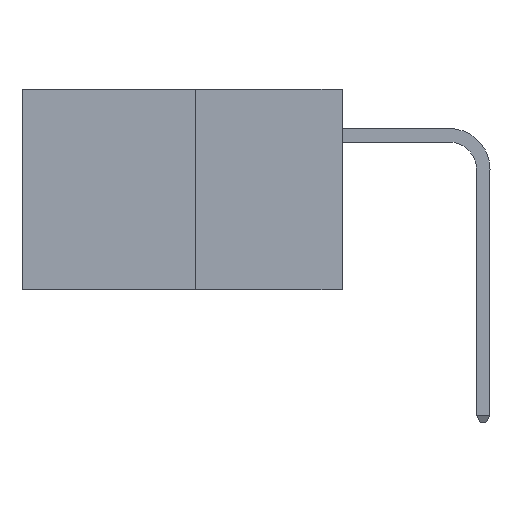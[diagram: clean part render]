
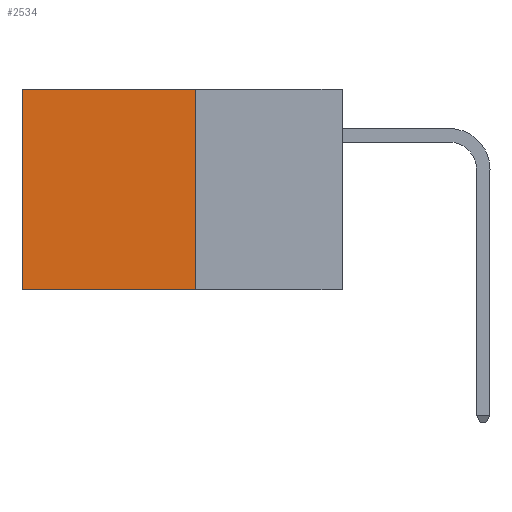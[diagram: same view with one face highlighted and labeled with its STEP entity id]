
A CAD part, left-side view. The second image highlights one B-rep face of the part: STEP entity #2534.
In plain terms, the highlighted planar face has unit normal (-1, 0, 0).
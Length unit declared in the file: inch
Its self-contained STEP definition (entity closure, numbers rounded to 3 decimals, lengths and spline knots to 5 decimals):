
#560 = EDGE_CURVE ( 'NONE', #17153, #22461, #20241, .T. ) ;
#880 = CARTESIAN_POINT ( 'NONE',  ( 0.277, 0.27, 0. ) ) ;
#1325 = VERTEX_POINT ( 'NONE', #22698 ) ;
#2214 = DIRECTION ( 'NONE',  ( 0., 0., -1. ) ) ;
#2436 = LINE ( 'NONE', #23840, #7656 ) ;
#2511 = DIRECTION ( 'NONE',  ( 1., 0., 0. ) ) ;
#2534 = ADVANCED_FACE ( 'NONE', ( #10246 ), #4251, .F. ) ;
#2813 = CARTESIAN_POINT ( 'NONE',  ( 0.277, 0.27, -0.37 ) ) ;
#4251 = PLANE ( 'NONE',  #25468 ) ;
#4839 = EDGE_LOOP ( 'NONE', ( #19494, #11584, #23456, #14546 ) ) ;
#6558 = DIRECTION ( 'NONE',  ( 0., 0., -1. ) ) ;
#6919 = CARTESIAN_POINT ( 'NONE',  ( 0.277, 0.27, -0.37 ) ) ;
#7656 = VECTOR ( 'NONE', #6558, 39.37008 ) ;
#7743 = EDGE_CURVE ( 'NONE', #8764, #17153, #15603, .T. ) ;
#8586 = EDGE_CURVE ( 'NONE', #8764, #1325, #2436, .T. ) ;
#8619 = VECTOR ( 'NONE', #23672, 39.37008 ) ;
#8764 = VERTEX_POINT ( 'NONE', #18065 ) ;
#9415 = EDGE_CURVE ( 'NONE', #1325, #22461, #21267, .T. ) ;
#10246 = FACE_OUTER_BOUND ( 'NONE', #4839, .T. ) ;
#11584 = ORIENTED_EDGE ( 'NONE', *, *, #9415, .F. ) ;
#12844 = VECTOR ( 'NONE', #20689, 39.37008 ) ;
#14546 = ORIENTED_EDGE ( 'NONE', *, *, #7743, .T. ) ;
#15603 = LINE ( 'NONE', #880, #12844 ) ;
#17128 = CARTESIAN_POINT ( 'NONE',  ( 0.277, 0.59, 0. ) ) ;
#17153 = VERTEX_POINT ( 'NONE', #17128 ) ;
#18065 = CARTESIAN_POINT ( 'NONE',  ( 0.277, 0.27, 0. ) ) ;
#19494 = ORIENTED_EDGE ( 'NONE', *, *, #560, .T. ) ;
#20241 = LINE ( 'NONE', #24576, #8619 ) ;
#20689 = DIRECTION ( 'NONE',  ( 0., 1., 0. ) ) ;
#21267 = LINE ( 'NONE', #6919, #27594 ) ;
#22461 = VERTEX_POINT ( 'NONE', #25406 ) ;
#22698 = CARTESIAN_POINT ( 'NONE',  ( 0.277, 0.27, -0.37 ) ) ;
#23456 = ORIENTED_EDGE ( 'NONE', *, *, #8586, .F. ) ;
#23672 = DIRECTION ( 'NONE',  ( 0., 0., -1. ) ) ;
#23840 = CARTESIAN_POINT ( 'NONE',  ( 0.277, 0.27, -0.37 ) ) ;
#24360 = DIRECTION ( 'NONE',  ( 0., 1., 0. ) ) ;
#24576 = CARTESIAN_POINT ( 'NONE',  ( 0.277, 0.59, -0.37 ) ) ;
#25406 = CARTESIAN_POINT ( 'NONE',  ( 0.277, 0.59, -0.37 ) ) ;
#25468 = AXIS2_PLACEMENT_3D ( 'NONE', #2813, #2511, #2214 ) ;
#27594 = VECTOR ( 'NONE', #24360, 39.37008 ) ;
